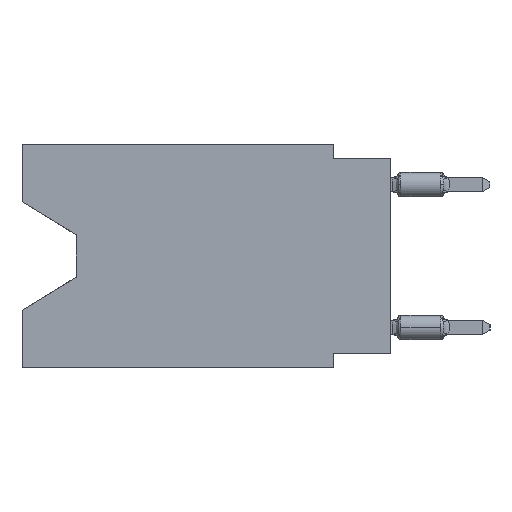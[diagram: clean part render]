
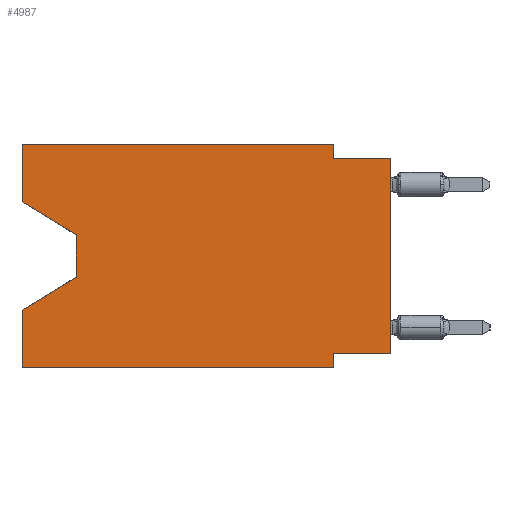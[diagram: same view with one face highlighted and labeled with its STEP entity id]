
A CAD part, left-side view. The second image highlights one B-rep face of the part: STEP entity #4987.
In plain terms, the highlighted planar face has unit normal (-1, 0, 0).
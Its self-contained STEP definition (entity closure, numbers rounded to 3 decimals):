
#945 = EDGE_CURVE ( 'NONE', #23012, #27190, #16611, .T. ) ;
#1352 = LINE ( 'NONE', #12725, #26409 ) ;
#1575 = DIRECTION ( 'NONE',  ( 0., -0.855, -0.519 ) ) ;
#2675 = EDGE_CURVE ( 'NONE', #23012, #17350, #15846, .T. ) ;
#2910 = EDGE_CURVE ( 'NONE', #30861, #8116, #12213, .T. ) ;
#3466 = VERTEX_POINT ( 'NONE', #17680 ) ;
#3568 = DIRECTION ( 'NONE',  ( 0., 0., 1. ) ) ;
#3819 = ORIENTED_EDGE ( 'NONE', *, *, #5128, .F. ) ;
#3861 = CARTESIAN_POINT ( 'NONE',  ( 0., 16.383, -9.906 ) ) ;
#3934 = EDGE_CURVE ( 'NONE', #4420, #27308, #24756, .T. ) ;
#4076 = DIRECTION ( 'NONE',  ( 0., 0., -1. ) ) ;
#4171 = ORIENTED_EDGE ( 'NONE', *, *, #2910, .T. ) ;
#4413 = DIRECTION ( 'NONE',  ( 0., 1., 0. ) ) ;
#4420 = VERTEX_POINT ( 'NONE', #28916 ) ;
#4987 = ADVANCED_FACE ( 'NONE', ( #12915 ), #10548, .F. ) ;
#5128 = EDGE_CURVE ( 'NONE', #17081, #6339, #20639, .T. ) ;
#5310 = CARTESIAN_POINT ( 'NONE',  ( 0., 16.383, 0. ) ) ;
#5508 = DIRECTION ( 'NONE',  ( 1., 0., 0. ) ) ;
#5828 = ORIENTED_EDGE ( 'NONE', *, *, #19660, .T. ) ;
#6339 = VERTEX_POINT ( 'NONE', #26418 ) ;
#6359 = LINE ( 'NONE', #16431, #24404 ) ;
#6620 = VECTOR ( 'NONE', #29467, 1000. ) ;
#6786 = CARTESIAN_POINT ( 'NONE',  ( 0., 0., -9.271 ) ) ;
#6997 = AXIS2_PLACEMENT_3D ( 'NONE', #20169, #5508, #15128 ) ;
#7937 = CARTESIAN_POINT ( 'NONE',  ( 0., 16.383, -9.906 ) ) ;
#8116 = VERTEX_POINT ( 'NONE', #21958 ) ;
#8296 = ORIENTED_EDGE ( 'NONE', *, *, #2675, .T. ) ;
#8423 = EDGE_CURVE ( 'NONE', #15903, #17622, #26036, .T. ) ;
#8456 = VECTOR ( 'NONE', #28169, 1000. ) ;
#9007 = EDGE_CURVE ( 'NONE', #17622, #17350, #14626, .T. ) ;
#9089 = VECTOR ( 'NONE', #4413, 1000. ) ;
#9519 = CARTESIAN_POINT ( 'NONE',  ( 0., 16.383, 0. ) ) ;
#9842 = DIRECTION ( 'NONE',  ( 0., 0., -1. ) ) ;
#9991 = ORIENTED_EDGE ( 'NONE', *, *, #9007, .F. ) ;
#10119 = EDGE_CURVE ( 'NONE', #4420, #30861, #20666, .T. ) ;
#10384 = CARTESIAN_POINT ( 'NONE',  ( 0., 16.383, 0. ) ) ;
#10548 = PLANE ( 'NONE',  #6997 ) ;
#10768 = VECTOR ( 'NONE', #14932, 1000. ) ;
#10941 = VECTOR ( 'NONE', #10956, 1000. ) ;
#10956 = DIRECTION ( 'NONE',  ( 0., -1., 0. ) ) ;
#11251 = CARTESIAN_POINT ( 'NONE',  ( 0., 0., -0.635 ) ) ;
#12213 = LINE ( 'NONE', #14571, #18993 ) ;
#12725 = CARTESIAN_POINT ( 'NONE',  ( 0., 0., 0. ) ) ;
#12915 = FACE_OUTER_BOUND ( 'NONE', #19681, .T. ) ;
#13582 = VECTOR ( 'NONE', #4076, 1000. ) ;
#14571 = CARTESIAN_POINT ( 'NONE',  ( 0., 13.97, -4.013 ) ) ;
#14626 = LINE ( 'NONE', #26942, #6620 ) ;
#14636 = VECTOR ( 'NONE', #20875, 1000. ) ;
#14932 = DIRECTION ( 'NONE',  ( 0., -1., 0. ) ) ;
#14946 = CARTESIAN_POINT ( 'NONE',  ( 0., 16.383, -7.36 ) ) ;
#15128 = DIRECTION ( 'NONE',  ( 0., 0., -1. ) ) ;
#15152 = EDGE_CURVE ( 'NONE', #6339, #3466, #30819, .T. ) ;
#15766 = CARTESIAN_POINT ( 'NONE',  ( 0., 16.383, -2.546 ) ) ;
#15846 = LINE ( 'NONE', #3861, #10941 ) ;
#15857 = CARTESIAN_POINT ( 'NONE',  ( 0., 13.97, -4.013 ) ) ;
#15903 = VERTEX_POINT ( 'NONE', #25819 ) ;
#15972 = DIRECTION ( 'NONE',  ( 0., 0.855, -0.519 ) ) ;
#16431 = CARTESIAN_POINT ( 'NONE',  ( 0., 13.97, -5.893 ) ) ;
#16611 = LINE ( 'NONE', #9519, #27512 ) ;
#17081 = VERTEX_POINT ( 'NONE', #24776 ) ;
#17350 = VERTEX_POINT ( 'NONE', #26634 ) ;
#17547 = ORIENTED_EDGE ( 'NONE', *, *, #20158, .T. ) ;
#17622 = VERTEX_POINT ( 'NONE', #26579 ) ;
#17680 = CARTESIAN_POINT ( 'NONE',  ( 0., 0., -0.635 ) ) ;
#18260 = CARTESIAN_POINT ( 'NONE',  ( 0., 2.54, 0. ) ) ;
#18993 = VECTOR ( 'NONE', #9842, 1000. ) ;
#19449 = ORIENTED_EDGE ( 'NONE', *, *, #8423, .F. ) ;
#19460 = EDGE_CURVE ( 'NONE', #27308, #17081, #19675, .T. ) ;
#19660 = EDGE_CURVE ( 'NONE', #15903, #3466, #1352, .T. ) ;
#19675 = LINE ( 'NONE', #5310, #10768 ) ;
#19681 = EDGE_LOOP ( 'NONE', ( #29128, #4171, #17547, #23176, #8296, #9991, #19449, #5828, #28067, #3819, #24020, #27301 ) ) ;
#20158 = EDGE_CURVE ( 'NONE', #8116, #27190, #6359, .T. ) ;
#20169 = CARTESIAN_POINT ( 'NONE',  ( 0., 16.383, 0. ) ) ;
#20639 = LINE ( 'NONE', #18260, #13582 ) ;
#20666 = LINE ( 'NONE', #15766, #28895 ) ;
#20774 = CARTESIAN_POINT ( 'NONE',  ( 0., 16.383, 0. ) ) ;
#20875 = DIRECTION ( 'NONE',  ( 0., -1., 0. ) ) ;
#21495 = DIRECTION ( 'NONE',  ( 0., 0., 1. ) ) ;
#21958 = CARTESIAN_POINT ( 'NONE',  ( 0., 13.97, -5.893 ) ) ;
#23012 = VERTEX_POINT ( 'NONE', #7937 ) ;
#23176 = ORIENTED_EDGE ( 'NONE', *, *, #945, .F. ) ;
#24020 = ORIENTED_EDGE ( 'NONE', *, *, #19460, .F. ) ;
#24404 = VECTOR ( 'NONE', #15972, 1000. ) ;
#24756 = LINE ( 'NONE', #10384, #8456 ) ;
#24776 = CARTESIAN_POINT ( 'NONE',  ( 0., 2.54, 0. ) ) ;
#25819 = CARTESIAN_POINT ( 'NONE',  ( 0., 0., -9.271 ) ) ;
#26036 = LINE ( 'NONE', #6786, #9089 ) ;
#26409 = VECTOR ( 'NONE', #3568, 1000. ) ;
#26418 = CARTESIAN_POINT ( 'NONE',  ( 0., 2.54, -0.635 ) ) ;
#26579 = CARTESIAN_POINT ( 'NONE',  ( 0., 2.54, -9.271 ) ) ;
#26634 = CARTESIAN_POINT ( 'NONE',  ( 0., 2.54, -9.906 ) ) ;
#26942 = CARTESIAN_POINT ( 'NONE',  ( 0., 2.54, -9.906 ) ) ;
#27190 = VERTEX_POINT ( 'NONE', #14946 ) ;
#27301 = ORIENTED_EDGE ( 'NONE', *, *, #3934, .F. ) ;
#27308 = VERTEX_POINT ( 'NONE', #20774 ) ;
#27512 = VECTOR ( 'NONE', #21495, 1000. ) ;
#28067 = ORIENTED_EDGE ( 'NONE', *, *, #15152, .F. ) ;
#28169 = DIRECTION ( 'NONE',  ( 0., 0., 1. ) ) ;
#28895 = VECTOR ( 'NONE', #1575, 1000. ) ;
#28916 = CARTESIAN_POINT ( 'NONE',  ( 0., 16.383, -2.546 ) ) ;
#29128 = ORIENTED_EDGE ( 'NONE', *, *, #10119, .T. ) ;
#29467 = DIRECTION ( 'NONE',  ( 0., 0., -1. ) ) ;
#30819 = LINE ( 'NONE', #11251, #14636 ) ;
#30861 = VERTEX_POINT ( 'NONE', #15857 ) ;
